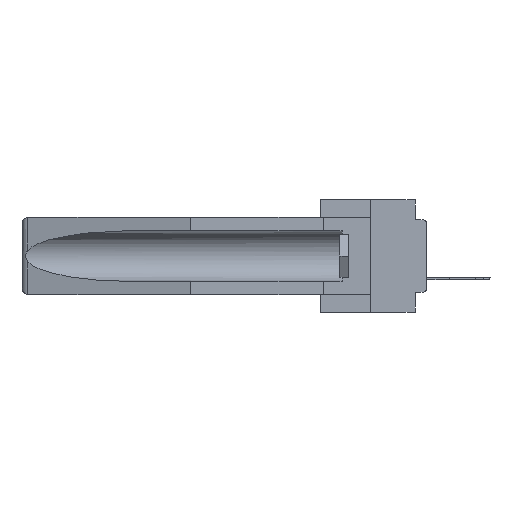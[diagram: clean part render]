
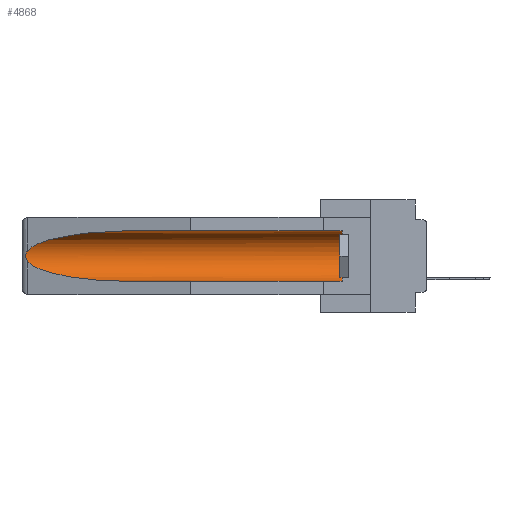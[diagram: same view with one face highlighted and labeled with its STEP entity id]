
A CAD part, left-side view. The second image highlights one B-rep face of the part: STEP entity #4868.
In plain terms, the highlighted cylindrical face has radius 2.857 mm (diameter 5.715 mm), a partial arc.
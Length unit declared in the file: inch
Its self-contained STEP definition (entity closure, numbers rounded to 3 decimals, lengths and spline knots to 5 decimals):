
#2353 = VERTEX_POINT ( 'NONE', #16283 ) ;
#2393 = CARTESIAN_POINT ( 'NONE',  ( 0.26537, 1.52718, -0.19328 ) ) ;
#3136 = CARTESIAN_POINT ( 'NONE',  ( 0.26537, 1.52718, -0.19328 ) ) ;
#3880 = CARTESIAN_POINT ( 'NONE',  ( 0.26537, 1.52718, -0.14972 ) ) ;
#4706 = CARTESIAN_POINT ( 'NONE',  ( 0.2675, 1.53308, -0.17534 ) ) ;
#4859 = CARTESIAN_POINT ( 'NONE',  ( 0.2673, 1.53269, -0.17917 ) ) ;
#4868 = ADVANCED_FACE ( 'NONE', ( #10816 ), #13590, .F. ) ;
#5739 = CARTESIAN_POINT ( 'NONE',  ( 0.21114, 1.30732, -0.284 ) ) ;
#5839 = DIRECTION ( 'NONE',  ( 0., -1., 0. ) ) ;
#6465 = ORIENTED_EDGE ( 'NONE', *, *, #10444, .T. ) ;
#6534 = EDGE_CURVE ( 'NONE', #12990, #29938, #18983, .T. ) ;
#7046 = CARTESIAN_POINT ( 'NONE',  ( 0.25451, 1.48313, -0.09465 ) ) ;
#7209 = CARTESIAN_POINT ( 'NONE',  ( 0.26537, 1.52718, -0.19328 ) ) ;
#7306 = CARTESIAN_POINT ( 'NONE',  ( 0.26597, 1.5296, -0.19026 ) ) ;
#7462 = CARTESIAN_POINT ( 'NONE',  ( 0.26655, 1.53094, -0.18657 ) ) ;
#8476 = CARTESIAN_POINT ( 'NONE',  ( 0.155, 1.07973, -0.059 ) ) ;
#8930 = VECTOR ( 'NONE', #9309, 39.37008 ) ;
#9309 = DIRECTION ( 'NONE',  ( 0., 1., 0. ) ) ;
#9599 = EDGE_CURVE ( 'NONE', #29938, #2353, #27204, .T. ) ;
#9859 = ORIENTED_EDGE ( 'NONE', *, *, #6534, .T. ) ;
#10044 = CARTESIAN_POINT ( 'NONE',  ( 0.155, 1.07973, -0.284 ) ) ;
#10444 = EDGE_CURVE ( 'NONE', #20425, #12990, #12497, .T. ) ;
#10816 = FACE_OUTER_BOUND ( 'NONE', #15446, .T. ) ;
#11046 = ORIENTED_EDGE ( 'NONE', *, *, #9599, .T. ) ;
#11380 = CARTESIAN_POINT ( 'NONE',  ( 0.155, 0.126, -0.059 ) ) ;
#11932 = CARTESIAN_POINT ( 'NONE',  ( 0.155, 0.126, -0.284 ) ) ;
#12497 =( BOUNDED_CURVE ( )  B_SPLINE_CURVE ( 3, ( #8476, #21043, #7046, #3880 ),
 .UNSPECIFIED., .F., .F. ) 
 B_SPLINE_CURVE_WITH_KNOTS ( ( 4, 4 ),
 ( 4.71239, 6.08839 ),
 .UNSPECIFIED. ) 
 CURVE ( )  GEOMETRIC_REPRESENTATION_ITEM ( )  RATIONAL_B_SPLINE_CURVE ( ( 1., 0.848, 0.848, 1. ) ) 
 REPRESENTATION_ITEM ( '' )  );
#12499 = ORIENTED_EDGE ( 'NONE', *, *, #23527, .F. ) ;
#12578 = AXIS2_PLACEMENT_3D ( 'NONE', #22127, #5839, #15220 ) ;
#12708 = VECTOR ( 'NONE', #30246, 39.37008 ) ;
#12990 = VERTEX_POINT ( 'NONE', #22140 ) ;
#13590 = CYLINDRICAL_SURFACE ( 'NONE', #25554, 0.1125 ) ;
#13811 = EDGE_CURVE ( 'NONE', #17039, #20425, #18691, .T. ) ;
#13942 = CARTESIAN_POINT ( 'NONE',  ( 0.155, -0.30754, -0.059 ) ) ;
#15220 = DIRECTION ( 'NONE',  ( 0., 0., 1. ) ) ;
#15446 = EDGE_LOOP ( 'NONE', ( #6465, #9859, #11046, #12499, #20418, #15690 ) ) ;
#15690 = ORIENTED_EDGE ( 'NONE', *, *, #13811, .T. ) ;
#16283 = CARTESIAN_POINT ( 'NONE',  ( 0.155, 1.07973, -0.284 ) ) ;
#16523 = CARTESIAN_POINT ( 'NONE',  ( 0.26654, 1.53092, -0.15636 ) ) ;
#17039 = VERTEX_POINT ( 'NONE', #11380 ) ;
#18691 = LINE ( 'NONE', #13942, #8930 ) ;
#18836 = CARTESIAN_POINT ( 'NONE',  ( 0.26537, 1.52718, -0.14972 ) ) ;
#18983 = B_SPLINE_CURVE_WITH_KNOTS ( 'NONE', 3,
 ( #18836, #25608, #16523, #23602, #28365, #4706, #4859, #7462, #7306, #2393 ),
 .UNSPECIFIED., .F., .F.,
 ( 4, 2, 2, 2, 4 ),
 ( 0., 0.00029, 0.00058, 0.00087, 0.00117 ),
 .UNSPECIFIED. ) ;
#19443 = CIRCLE ( 'NONE', #12578, 0.1125 ) ;
#20209 = DIRECTION ( 'NONE',  ( 0., 1., 0. ) ) ;
#20418 = ORIENTED_EDGE ( 'NONE', *, *, #20609, .T. ) ;
#20425 = VERTEX_POINT ( 'NONE', #26431 ) ;
#20609 = EDGE_CURVE ( 'NONE', #25175, #17039, #19443, .T. ) ;
#20867 = LINE ( 'NONE', #28234, #12708 ) ;
#21043 = CARTESIAN_POINT ( 'NONE',  ( 0.21114, 1.30732, -0.059 ) ) ;
#22127 = CARTESIAN_POINT ( 'NONE',  ( 0.155, 0.126, -0.1715 ) ) ;
#22140 = CARTESIAN_POINT ( 'NONE',  ( 0.26537, 1.52718, -0.14972 ) ) ;
#22958 = CARTESIAN_POINT ( 'NONE',  ( 0.155, -0.30754, -0.1715 ) ) ;
#23527 = EDGE_CURVE ( 'NONE', #25175, #2353, #20867, .T. ) ;
#23602 = CARTESIAN_POINT ( 'NONE',  ( 0.2673, 1.5327, -0.16383 ) ) ;
#25175 = VERTEX_POINT ( 'NONE', #11932 ) ;
#25554 = AXIS2_PLACEMENT_3D ( 'NONE', #22958, #20209, #29585 ) ;
#25608 = CARTESIAN_POINT ( 'NONE',  ( 0.26597, 1.52961, -0.15275 ) ) ;
#26431 = CARTESIAN_POINT ( 'NONE',  ( 0.155, 1.07973, -0.059 ) ) ;
#26482 = CARTESIAN_POINT ( 'NONE',  ( 0.25451, 1.48313, -0.24835 ) ) ;
#27204 =( BOUNDED_CURVE ( )  B_SPLINE_CURVE ( 3, ( #3136, #26482, #5739, #10044 ),
 .UNSPECIFIED., .F., .F. ) 
 B_SPLINE_CURVE_WITH_KNOTS ( ( 4, 4 ),
 ( 0.1948, 1.5708 ),
 .UNSPECIFIED. ) 
 CURVE ( )  GEOMETRIC_REPRESENTATION_ITEM ( )  RATIONAL_B_SPLINE_CURVE ( ( 1., 0.848, 0.848, 1. ) ) 
 REPRESENTATION_ITEM ( '' )  );
#28234 = CARTESIAN_POINT ( 'NONE',  ( 0.155, -0.30754, -0.284 ) ) ;
#28365 = CARTESIAN_POINT ( 'NONE',  ( 0.2675, 1.53308, -0.16763 ) ) ;
#29585 = DIRECTION ( 'NONE',  ( 0., 0., 1. ) ) ;
#29938 = VERTEX_POINT ( 'NONE', #7209 ) ;
#30246 = DIRECTION ( 'NONE',  ( 0., 1., 0. ) ) ;
